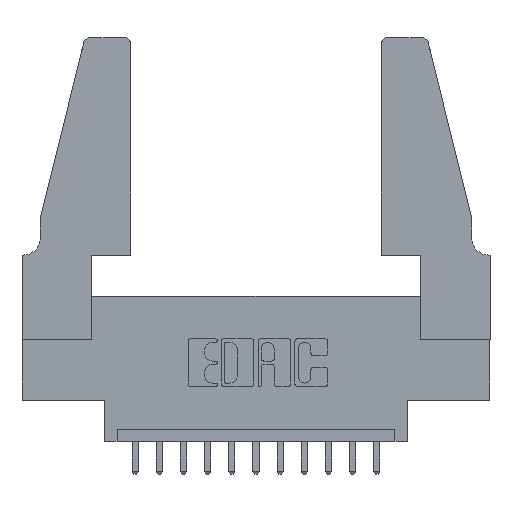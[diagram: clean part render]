
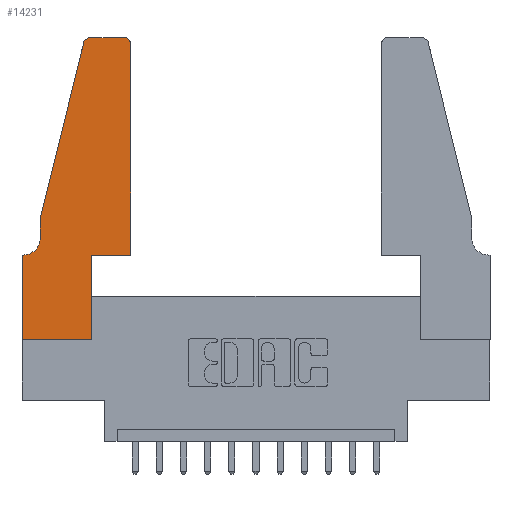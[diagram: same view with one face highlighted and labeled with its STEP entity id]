
A CAD part, top view. The second image highlights one B-rep face of the part: STEP entity #14231.
In plain terms, the highlighted planar face has unit normal (0, 0, 1).
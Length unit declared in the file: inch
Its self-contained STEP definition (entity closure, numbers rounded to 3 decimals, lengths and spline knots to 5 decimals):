
#33 = CARTESIAN_POINT ( 'NONE',  ( 0.2865, 0.35, 0.37 ) ) ;
#378 = CARTESIAN_POINT ( 'NONE',  ( 0., 0., 0.37 ) ) ;
#385 = AXIS2_PLACEMENT_3D ( 'NONE', #10764, #12020, #6172 ) ;
#418 = VERTEX_POINT ( 'NONE', #10781 ) ;
#453 = CARTESIAN_POINT ( 'NONE',  ( 0., 0.35, 0.37 ) ) ;
#1457 = VECTOR ( 'NONE', #14148, 39.37008 ) ;
#1549 = LINE ( 'NONE', #13512, #4426 ) ;
#1822 = CARTESIAN_POINT ( 'NONE',  ( 0.0755, 0.5, 0.37 ) ) ;
#2119 = CARTESIAN_POINT ( 'NONE',  ( 0., 0.35, 0.37 ) ) ;
#2202 = FACE_OUTER_BOUND ( 'NONE', #10503, .T. ) ;
#2636 = CARTESIAN_POINT ( 'NONE',  ( 0.0755, 0.42, 0.37 ) ) ;
#2910 = CARTESIAN_POINT ( 'NONE',  ( 0.2865, 0.35, 0.37 ) ) ;
#2911 = DIRECTION ( 'NONE',  ( -0.239, -0.971, 0. ) ) ;
#3140 = EDGE_CURVE ( 'NONE', #7350, #7627, #14474, .T. ) ;
#3250 = ORIENTED_EDGE ( 'NONE', *, *, #3447, .T. ) ;
#3311 = ORIENTED_EDGE ( 'NONE', *, *, #8024, .T. ) ;
#3447 = EDGE_CURVE ( 'NONE', #13293, #14171, #6444, .T. ) ;
#3455 = VECTOR ( 'NONE', #6966, 39.37008 ) ;
#3576 = CARTESIAN_POINT ( 'NONE',  ( 0.4505, 1.22, 0.37 ) ) ;
#3580 = CIRCLE ( 'NONE', #3648, 0.03 ) ;
#3648 = AXIS2_PLACEMENT_3D ( 'NONE', #14721, #7828, #6634 ) ;
#4067 = CARTESIAN_POINT ( 'NONE',  ( 0.2605, 1.25, 0.37 ) ) ;
#4426 = VECTOR ( 'NONE', #5457, 39.37008 ) ;
#4918 = CIRCLE ( 'NONE', #385, 0.03 ) ;
#5073 = VERTEX_POINT ( 'NONE', #3576 ) ;
#5453 = ORIENTED_EDGE ( 'NONE', *, *, #7876, .T. ) ;
#5457 = DIRECTION ( 'NONE',  ( 0., 1., 0. ) ) ;
#5967 = LINE ( 'NONE', #12943, #1457 ) ;
#5980 = ORIENTED_EDGE ( 'NONE', *, *, #14564, .T. ) ;
#6172 = DIRECTION ( 'NONE',  ( 1., 0., 0. ) ) ;
#6184 = ORIENTED_EDGE ( 'NONE', *, *, #8509, .T. ) ;
#6340 = EDGE_CURVE ( 'NONE', #14115, #13586, #10100, .T. ) ;
#6444 = LINE ( 'NONE', #33, #10190 ) ;
#6501 = VERTEX_POINT ( 'NONE', #378 ) ;
#6634 = DIRECTION ( 'NONE',  ( 1., 0., 0. ) ) ;
#6658 = DIRECTION ( 'NONE',  ( 1., 0., 0. ) ) ;
#6729 = EDGE_CURVE ( 'NONE', #14134, #7350, #3580, .T. ) ;
#6966 = DIRECTION ( 'NONE',  ( 1., 0., 0. ) ) ;
#7134 = VECTOR ( 'NONE', #9922, 39.37008 ) ;
#7326 = EDGE_CURVE ( 'NONE', #418, #5073, #1549, .T. ) ;
#7350 = VERTEX_POINT ( 'NONE', #11143 ) ;
#7386 = CARTESIAN_POINT ( 'NONE',  ( 0.4205, 1.25, 0.37 ) ) ;
#7627 = VERTEX_POINT ( 'NONE', #9482 ) ;
#7828 = DIRECTION ( 'NONE',  ( 0., 0., 1. ) ) ;
#7850 = DIRECTION ( 'NONE',  ( 0., 1., 0. ) ) ;
#7876 = EDGE_CURVE ( 'NONE', #12733, #14115, #8561, .T. ) ;
#7945 = PLANE ( 'NONE',  #14400 ) ;
#7947 = DIRECTION ( 'NONE',  ( -1., 0., 0. ) ) ;
#8024 = EDGE_CURVE ( 'NONE', #14659, #14134, #13863, .T. ) ;
#8509 = EDGE_CURVE ( 'NONE', #5073, #14659, #4918, .T. ) ;
#8561 = CIRCLE ( 'NONE', #8642, 0.07 ) ;
#8642 = AXIS2_PLACEMENT_3D ( 'NONE', #9717, #12867, #11955 ) ;
#8717 = CARTESIAN_POINT ( 'NONE',  ( 0.284, 1.25, 0.37 ) ) ;
#8959 = ORIENTED_EDGE ( 'NONE', *, *, #7326, .T. ) ;
#9071 = DIRECTION ( 'NONE',  ( 0., 0., 1. ) ) ;
#9482 = CARTESIAN_POINT ( 'NONE',  ( 0.0755, 0.5, 0.37 ) ) ;
#9486 = LINE ( 'NONE', #10819, #9852 ) ;
#9582 = ORIENTED_EDGE ( 'NONE', *, *, #6729, .T. ) ;
#9670 = ORIENTED_EDGE ( 'NONE', *, *, #13683, .T. ) ;
#9717 = CARTESIAN_POINT ( 'NONE',  ( 0.0055, 0.42, 0.37 ) ) ;
#9764 = ORIENTED_EDGE ( 'NONE', *, *, #12779, .T. ) ;
#9815 = CARTESIAN_POINT ( 'NONE',  ( 0., 0., 0.37 ) ) ;
#9852 = VECTOR ( 'NONE', #10623, 39.37008 ) ;
#9922 = DIRECTION ( 'NONE',  ( -1., 0., 0. ) ) ;
#10100 = LINE ( 'NONE', #12606, #10804 ) ;
#10190 = VECTOR ( 'NONE', #7850, 39.37008 ) ;
#10503 = EDGE_LOOP ( 'NONE', ( #3311, #9582, #11373, #5980, #5453, #12329, #9764, #9670, #3250, #11194, #8959, #6184 ) ) ;
#10562 = VECTOR ( 'NONE', #12809, 39.37008 ) ;
#10623 = DIRECTION ( 'NONE',  ( 0., -1., 0. ) ) ;
#10764 = CARTESIAN_POINT ( 'NONE',  ( 0.4205, 1.22, 0.37 ) ) ;
#10781 = CARTESIAN_POINT ( 'NONE',  ( 0.4505, 0.35, 0.37 ) ) ;
#10804 = VECTOR ( 'NONE', #7947, 39.37008 ) ;
#10819 = CARTESIAN_POINT ( 'NONE',  ( 0., 0., 0.37 ) ) ;
#11143 = CARTESIAN_POINT ( 'NONE',  ( 0.25487, 1.22718, 0.37 ) ) ;
#11194 = ORIENTED_EDGE ( 'NONE', *, *, #11540, .T. ) ;
#11373 = ORIENTED_EDGE ( 'NONE', *, *, #3140, .T. ) ;
#11540 = EDGE_CURVE ( 'NONE', #14171, #418, #13564, .T. ) ;
#11643 = CARTESIAN_POINT ( 'NONE',  ( 0.4505, 0.35, 0.37 ) ) ;
#11955 = DIRECTION ( 'NONE',  ( -1., 0., 0. ) ) ;
#12020 = DIRECTION ( 'NONE',  ( 0., 0., 1. ) ) ;
#12143 = CARTESIAN_POINT ( 'NONE',  ( 0.0055, 0.35, 0.37 ) ) ;
#12329 = ORIENTED_EDGE ( 'NONE', *, *, #6340, .T. ) ;
#12606 = CARTESIAN_POINT ( 'NONE',  ( 0.0755, 0.35, 0.37 ) ) ;
#12733 = VERTEX_POINT ( 'NONE', #2636 ) ;
#12779 = EDGE_CURVE ( 'NONE', #13586, #6501, #9486, .T. ) ;
#12809 = DIRECTION ( 'NONE',  ( 1., 0., 0. ) ) ;
#12867 = DIRECTION ( 'NONE',  ( 0., 0., -1. ) ) ;
#12943 = CARTESIAN_POINT ( 'NONE',  ( 0.0755, 0.5, 0.37 ) ) ;
#13293 = VERTEX_POINT ( 'NONE', #14768 ) ;
#13374 = VECTOR ( 'NONE', #2911, 39.37008 ) ;
#13473 = LINE ( 'NONE', #9815, #3455 ) ;
#13512 = CARTESIAN_POINT ( 'NONE',  ( 0.4505, 0.35, 0.37 ) ) ;
#13564 = LINE ( 'NONE', #11643, #10562 ) ;
#13586 = VERTEX_POINT ( 'NONE', #453 ) ;
#13683 = EDGE_CURVE ( 'NONE', #6501, #13293, #13473, .T. ) ;
#13863 = LINE ( 'NONE', #4067, #7134 ) ;
#14115 = VERTEX_POINT ( 'NONE', #12143 ) ;
#14134 = VERTEX_POINT ( 'NONE', #8717 ) ;
#14148 = DIRECTION ( 'NONE',  ( 0., -1., 0. ) ) ;
#14171 = VERTEX_POINT ( 'NONE', #2910 ) ;
#14231 = ADVANCED_FACE ( 'NONE', ( #2202 ), #7945, .T. ) ;
#14400 = AXIS2_PLACEMENT_3D ( 'NONE', #2119, #9071, #6658 ) ;
#14474 = LINE ( 'NONE', #1822, #13374 ) ;
#14564 = EDGE_CURVE ( 'NONE', #7627, #12733, #5967, .T. ) ;
#14659 = VERTEX_POINT ( 'NONE', #7386 ) ;
#14721 = CARTESIAN_POINT ( 'NONE',  ( 0.284, 1.22, 0.37 ) ) ;
#14768 = CARTESIAN_POINT ( 'NONE',  ( 0.2865, 0., 0.37 ) ) ;
